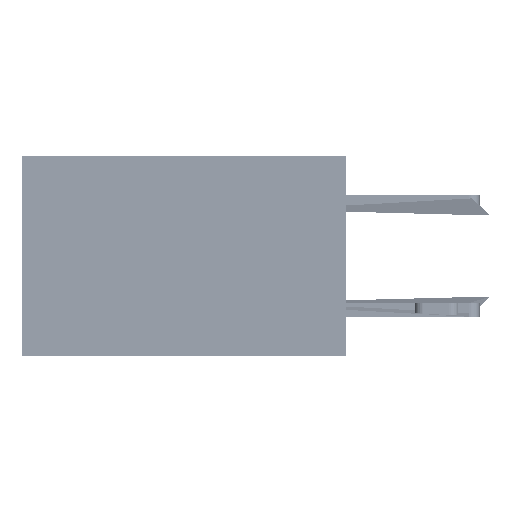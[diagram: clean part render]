
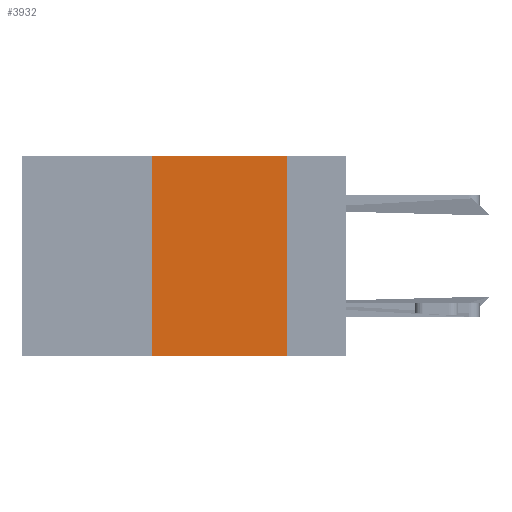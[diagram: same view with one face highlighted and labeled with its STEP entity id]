
A CAD part, left-side view. The second image highlights one B-rep face of the part: STEP entity #3932.
In plain terms, the highlighted planar face has unit normal (-1, 0, 0).
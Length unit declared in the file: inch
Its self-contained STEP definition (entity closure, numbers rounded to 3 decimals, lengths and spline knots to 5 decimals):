
#1034 = CARTESIAN_POINT ( 'NONE',  ( 0., 0.6, -0.37 ) ) ;
#1371 = DIRECTION ( 'NONE',  ( 0., -1., 0. ) ) ;
#1985 = VERTEX_POINT ( 'NONE', #15395 ) ;
#3932 = ADVANCED_FACE ( 'NONE', ( #13125 ), #18015, .F. ) ;
#4481 = LINE ( 'NONE', #48976, #27062 ) ;
#5098 = LINE ( 'NONE', #1034, #8896 ) ;
#5277 = CARTESIAN_POINT ( 'NONE',  ( 0., 0.36, 0. ) ) ;
#5621 = VERTEX_POINT ( 'NONE', #44628 ) ;
#5642 = EDGE_CURVE ( 'NONE', #19231, #48044, #35563, .T. ) ;
#8242 = EDGE_CURVE ( 'NONE', #48044, #5621, #4481, .T. ) ;
#8896 = VECTOR ( 'NONE', #1371, 39.37008 ) ;
#9055 = DIRECTION ( 'NONE',  ( 0., -1., 0. ) ) ;
#9153 = CARTESIAN_POINT ( 'NONE',  ( 0., 0.11, 0. ) ) ;
#10144 = DIRECTION ( 'NONE',  ( 1., 0., 0. ) ) ;
#10677 = CARTESIAN_POINT ( 'NONE',  ( 0., 0.36, -0.37 ) ) ;
#10831 = AXIS2_PLACEMENT_3D ( 'NONE', #45873, #10144, #46046 ) ;
#11408 = ORIENTED_EDGE ( 'NONE', *, *, #8242, .F. ) ;
#12832 = CARTESIAN_POINT ( 'NONE',  ( 0., 0.36, 0. ) ) ;
#13125 = FACE_OUTER_BOUND ( 'NONE', #32883, .T. ) ;
#13250 = LINE ( 'NONE', #9153, #48365 ) ;
#15395 = CARTESIAN_POINT ( 'NONE',  ( 0., 0.11, -0.37 ) ) ;
#18015 = PLANE ( 'NONE',  #10831 ) ;
#19231 = VERTEX_POINT ( 'NONE', #10677 ) ;
#20877 = ORIENTED_EDGE ( 'NONE', *, *, #5642, .F. ) ;
#24507 = ORIENTED_EDGE ( 'NONE', *, *, #29460, .T. ) ;
#27062 = VECTOR ( 'NONE', #9055, 39.37008 ) ;
#29460 = EDGE_CURVE ( 'NONE', #19231, #1985, #5098, .T. ) ;
#30068 = ORIENTED_EDGE ( 'NONE', *, *, #49925, .F. ) ;
#32883 = EDGE_LOOP ( 'NONE', ( #30068, #11408, #20877, #24507 ) ) ;
#35563 = LINE ( 'NONE', #5277, #37422 ) ;
#37422 = VECTOR ( 'NONE', #49425, 39.37008 ) ;
#37522 = DIRECTION ( 'NONE',  ( 0., 0., -1. ) ) ;
#44628 = CARTESIAN_POINT ( 'NONE',  ( 0., 0.11, 0. ) ) ;
#45873 = CARTESIAN_POINT ( 'NONE',  ( 0., 0.6, 0. ) ) ;
#46046 = DIRECTION ( 'NONE',  ( 0., 0., -1. ) ) ;
#48044 = VERTEX_POINT ( 'NONE', #12832 ) ;
#48365 = VECTOR ( 'NONE', #37522, 39.37008 ) ;
#48976 = CARTESIAN_POINT ( 'NONE',  ( 0., 0.6, 0. ) ) ;
#49425 = DIRECTION ( 'NONE',  ( 0., 0., 1. ) ) ;
#49925 = EDGE_CURVE ( 'NONE', #5621, #1985, #13250, .T. ) ;
